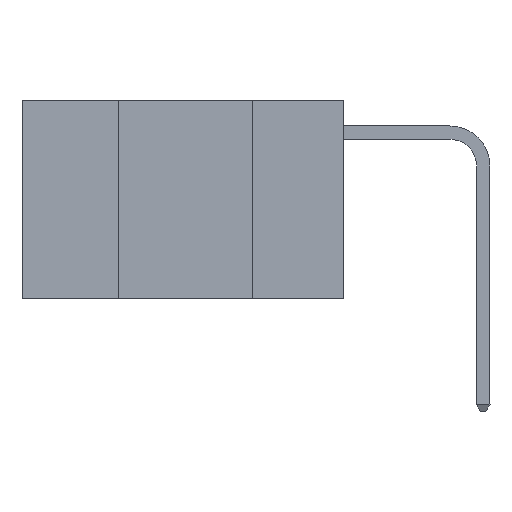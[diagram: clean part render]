
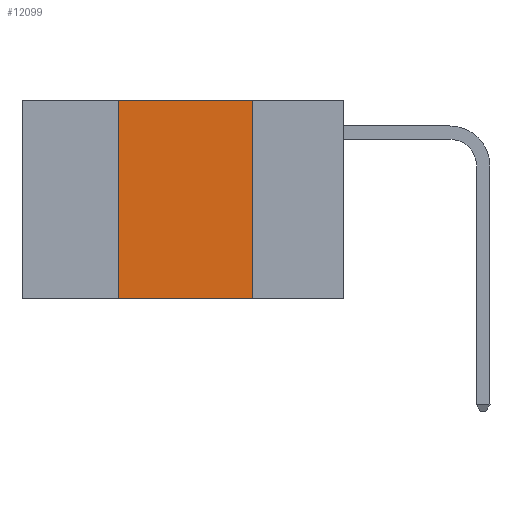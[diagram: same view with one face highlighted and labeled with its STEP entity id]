
A CAD part, left-side view. The second image highlights one B-rep face of the part: STEP entity #12099.
In plain terms, the highlighted planar face has unit normal (-1, 0, 0).
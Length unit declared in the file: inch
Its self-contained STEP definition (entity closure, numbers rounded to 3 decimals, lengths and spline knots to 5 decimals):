
#114 = VERTEX_POINT ( 'NONE', #14438 ) ;
#568 = CARTESIAN_POINT ( 'NONE',  ( 0., 0.42, -0.37 ) ) ;
#823 = EDGE_LOOP ( 'NONE', ( #13427, #15932, #7425, #6698 ) ) ;
#841 = FACE_OUTER_BOUND ( 'NONE', #823, .T. ) ;
#1055 = VECTOR ( 'NONE', #17203, 39.37008 ) ;
#1467 = LINE ( 'NONE', #3171, #9355 ) ;
#2652 = PLANE ( 'NONE',  #22246 ) ;
#2759 = DIRECTION ( 'NONE',  ( 0., 0., -1. ) ) ;
#3171 = CARTESIAN_POINT ( 'NONE',  ( 0., 0.6, 0. ) ) ;
#3935 = VECTOR ( 'NONE', #18802, 39.37008 ) ;
#4383 = CARTESIAN_POINT ( 'NONE',  ( 0., 0.6, -0.37 ) ) ;
#4473 = DIRECTION ( 'NONE',  ( 1., 0., 0. ) ) ;
#5100 = LINE ( 'NONE', #9926, #5169 ) ;
#5150 = VERTEX_POINT ( 'NONE', #568 ) ;
#5169 = VECTOR ( 'NONE', #11967, 39.37008 ) ;
#6698 = ORIENTED_EDGE ( 'NONE', *, *, #11562, .T. ) ;
#7425 = ORIENTED_EDGE ( 'NONE', *, *, #22219, .F. ) ;
#7576 = VERTEX_POINT ( 'NONE', #15582 ) ;
#7908 = CARTESIAN_POINT ( 'NONE',  ( 0., 0.6, 0. ) ) ;
#8916 = VERTEX_POINT ( 'NONE', #21540 ) ;
#9355 = VECTOR ( 'NONE', #22191, 39.37008 ) ;
#9476 = EDGE_CURVE ( 'NONE', #8916, #7576, #1467, .T. ) ;
#9926 = CARTESIAN_POINT ( 'NONE',  ( 0., 0.42, 0. ) ) ;
#11562 = EDGE_CURVE ( 'NONE', #5150, #114, #14904, .T. ) ;
#11967 = DIRECTION ( 'NONE',  ( 0., 0., 1. ) ) ;
#12099 = ADVANCED_FACE ( 'NONE', ( #841 ), #2652, .F. ) ;
#13427 = ORIENTED_EDGE ( 'NONE', *, *, #13792, .F. ) ;
#13792 = EDGE_CURVE ( 'NONE', #7576, #114, #17433, .T. ) ;
#14438 = CARTESIAN_POINT ( 'NONE',  ( 0., 0.17, -0.37 ) ) ;
#14904 = LINE ( 'NONE', #4383, #3935 ) ;
#15582 = CARTESIAN_POINT ( 'NONE',  ( 0., 0.17, 0. ) ) ;
#15932 = ORIENTED_EDGE ( 'NONE', *, *, #9476, .F. ) ;
#17203 = DIRECTION ( 'NONE',  ( 0., 0., -1. ) ) ;
#17433 = LINE ( 'NONE', #20878, #1055 ) ;
#18802 = DIRECTION ( 'NONE',  ( 0., -1., 0. ) ) ;
#20878 = CARTESIAN_POINT ( 'NONE',  ( 0., 0.17, 0. ) ) ;
#21540 = CARTESIAN_POINT ( 'NONE',  ( 0., 0.42, 0. ) ) ;
#22191 = DIRECTION ( 'NONE',  ( 0., -1., 0. ) ) ;
#22219 = EDGE_CURVE ( 'NONE', #5150, #8916, #5100, .T. ) ;
#22246 = AXIS2_PLACEMENT_3D ( 'NONE', #7908, #4473, #2759 ) ;
